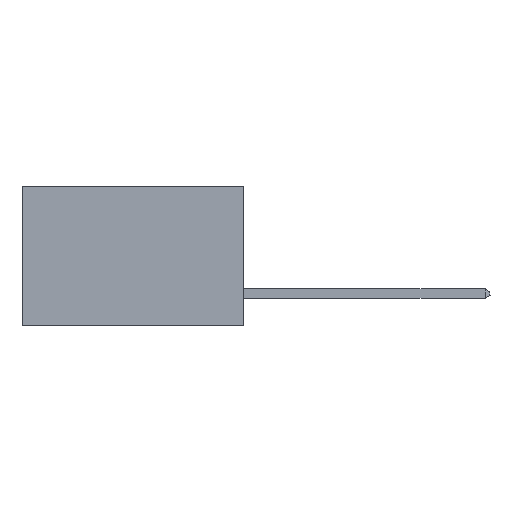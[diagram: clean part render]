
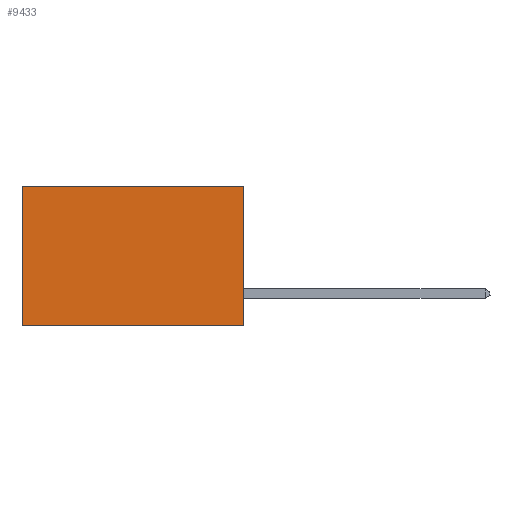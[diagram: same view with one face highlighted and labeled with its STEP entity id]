
A CAD part, left-side view. The second image highlights one B-rep face of the part: STEP entity #9433.
In plain terms, the highlighted planar face has unit normal (-1, 0, 0).
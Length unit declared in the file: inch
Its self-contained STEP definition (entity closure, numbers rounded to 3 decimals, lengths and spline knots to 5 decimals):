
#3030 = LINE ( 'NONE', #27165, #25524 ) ;
#3343 = CARTESIAN_POINT ( 'NONE',  ( 0.277, 0.59, 0. ) ) ;
#3607 = CARTESIAN_POINT ( 'NONE',  ( 0.277, 0., 0. ) ) ;
#5606 = VERTEX_POINT ( 'NONE', #27925 ) ;
#5613 = LINE ( 'NONE', #20847, #10828 ) ;
#5944 = VERTEX_POINT ( 'NONE', #24512 ) ;
#6564 = CARTESIAN_POINT ( 'NONE',  ( 0.277, 0., -0.37 ) ) ;
#6827 = DIRECTION ( 'NONE',  ( 0., 0., -1. ) ) ;
#7162 = EDGE_LOOP ( 'NONE', ( #13669, #19881, #17412, #19813 ) ) ;
#7348 = EDGE_CURVE ( 'NONE', #8201, #5606, #5613, .T. ) ;
#8201 = VERTEX_POINT ( 'NONE', #3607 ) ;
#8812 = DIRECTION ( 'NONE',  ( 1., 0., 0. ) ) ;
#9433 = ADVANCED_FACE ( 'NONE', ( #12753 ), #21859, .F. ) ;
#9794 = EDGE_CURVE ( 'NONE', #8201, #11049, #3030, .T. ) ;
#9885 = DIRECTION ( 'NONE',  ( 0., 1., 0. ) ) ;
#10438 = EDGE_CURVE ( 'NONE', #5606, #5944, #20777, .T. ) ;
#10828 = VECTOR ( 'NONE', #20685, 39.37008 ) ;
#11049 = VERTEX_POINT ( 'NONE', #3343 ) ;
#12064 = DIRECTION ( 'NONE',  ( 0., 1., 0. ) ) ;
#12753 = FACE_OUTER_BOUND ( 'NONE', #7162, .T. ) ;
#13445 = CARTESIAN_POINT ( 'NONE',  ( 0.277, 0.59, -0.37 ) ) ;
#13669 = ORIENTED_EDGE ( 'NONE', *, *, #23222, .T. ) ;
#15527 = AXIS2_PLACEMENT_3D ( 'NONE', #6564, #8812, #24000 ) ;
#17412 = ORIENTED_EDGE ( 'NONE', *, *, #7348, .F. ) ;
#19813 = ORIENTED_EDGE ( 'NONE', *, *, #9794, .T. ) ;
#19881 = ORIENTED_EDGE ( 'NONE', *, *, #10438, .F. ) ;
#20685 = DIRECTION ( 'NONE',  ( 0., 0., -1. ) ) ;
#20777 = LINE ( 'NONE', #24977, #21435 ) ;
#20847 = CARTESIAN_POINT ( 'NONE',  ( 0.277, 0., -0.37 ) ) ;
#21435 = VECTOR ( 'NONE', #12064, 39.37008 ) ;
#21859 = PLANE ( 'NONE',  #15527 ) ;
#23222 = EDGE_CURVE ( 'NONE', #11049, #5944, #27143, .T. ) ;
#24000 = DIRECTION ( 'NONE',  ( 0., 0., -1. ) ) ;
#24512 = CARTESIAN_POINT ( 'NONE',  ( 0.277, 0.59, -0.37 ) ) ;
#24977 = CARTESIAN_POINT ( 'NONE',  ( 0.277, 0., -0.37 ) ) ;
#25524 = VECTOR ( 'NONE', #9885, 39.37008 ) ;
#25814 = VECTOR ( 'NONE', #6827, 39.37008 ) ;
#27143 = LINE ( 'NONE', #13445, #25814 ) ;
#27165 = CARTESIAN_POINT ( 'NONE',  ( 0.277, 0., 0. ) ) ;
#27925 = CARTESIAN_POINT ( 'NONE',  ( 0.277, 0., -0.37 ) ) ;
